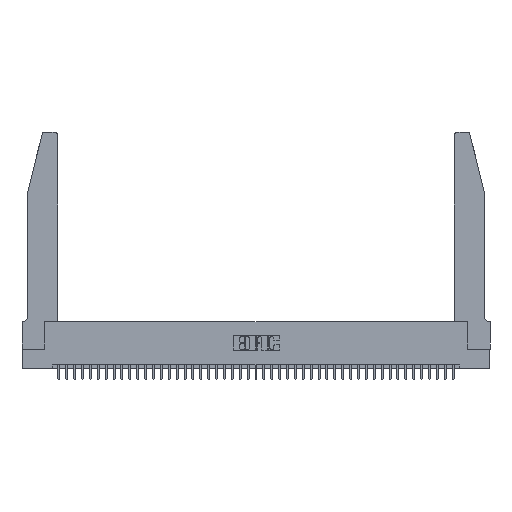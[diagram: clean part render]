
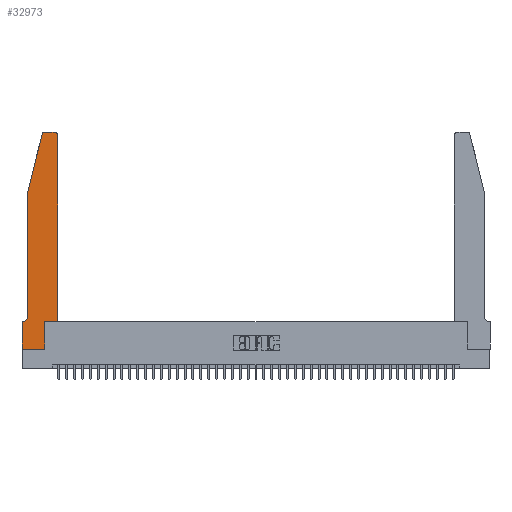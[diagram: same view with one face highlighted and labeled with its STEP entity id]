
A CAD part, top view. The second image highlights one B-rep face of the part: STEP entity #32973.
In plain terms, the highlighted planar face has unit normal (0, 0, 1).
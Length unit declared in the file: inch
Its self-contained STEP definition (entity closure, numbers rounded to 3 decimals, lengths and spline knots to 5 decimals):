
#164 = ORIENTED_EDGE ( 'NONE', *, *, #26499, .T. ) ;
#203 = ORIENTED_EDGE ( 'NONE', *, *, #35338, .T. ) ;
#878 = VERTEX_POINT ( 'NONE', #36373 ) ;
#2096 = LINE ( 'NONE', #17351, #25186 ) ;
#2854 = CARTESIAN_POINT ( 'NONE',  ( 0., 0.35, 0.37 ) ) ;
#3001 = VECTOR ( 'NONE', #38854, 39.37008 ) ;
#3074 = CARTESIAN_POINT ( 'NONE',  ( 0.2865, 0.35, 0.37 ) ) ;
#3281 = EDGE_CURVE ( 'NONE', #15961, #9850, #2096, .T. ) ;
#3304 = CARTESIAN_POINT ( 'NONE',  ( 0.0055, 0.42, 0.37 ) ) ;
#3636 = DIRECTION ( 'NONE',  ( -1., 0., 0. ) ) ;
#3750 = CARTESIAN_POINT ( 'NONE',  ( 0.4505, 0.35, 0.37 ) ) ;
#4304 = VERTEX_POINT ( 'NONE', #29953 ) ;
#4739 = DIRECTION ( 'NONE',  ( -0.239, -0.971, 0. ) ) ;
#4742 = DIRECTION ( 'NONE',  ( 1., 0., 0. ) ) ;
#5347 = DIRECTION ( 'NONE',  ( 0., 0., 1. ) ) ;
#5674 = VERTEX_POINT ( 'NONE', #12867 ) ;
#6853 = ORIENTED_EDGE ( 'NONE', *, *, #35453, .T. ) ;
#6986 = CARTESIAN_POINT ( 'NONE',  ( 0.0755, 0.35, 0.37 ) ) ;
#7164 = CARTESIAN_POINT ( 'NONE',  ( 0.0055, 0.35, 0.37 ) ) ;
#7631 = DIRECTION ( 'NONE',  ( 0., 0., 1. ) ) ;
#7651 = ORIENTED_EDGE ( 'NONE', *, *, #23992, .T. ) ;
#7680 = CIRCLE ( 'NONE', #9262, 0.07 ) ;
#8146 = EDGE_LOOP ( 'NONE', ( #14916, #164, #42248, #7651, #203, #36107, #33491, #30546, #33641, #6853, #37610, #27433 ) ) ;
#8549 = CIRCLE ( 'NONE', #38478, 0.03 ) ;
#9124 = EDGE_CURVE ( 'NONE', #31547, #4304, #24415, .T. ) ;
#9262 = AXIS2_PLACEMENT_3D ( 'NONE', #3304, #26938, #19879 ) ;
#9484 = PLANE ( 'NONE',  #35426 ) ;
#9835 = VECTOR ( 'NONE', #3636, 39.37008 ) ;
#9850 = VERTEX_POINT ( 'NONE', #31235 ) ;
#11353 = LINE ( 'NONE', #6986, #9835 ) ;
#11433 = EDGE_CURVE ( 'NONE', #878, #14352, #15251, .T. ) ;
#11893 = VECTOR ( 'NONE', #27755, 39.37008 ) ;
#12841 = DIRECTION ( 'NONE',  ( 1., 0., 0. ) ) ;
#12867 = CARTESIAN_POINT ( 'NONE',  ( 0.4205, 2.75, 0.37 ) ) ;
#13540 = VERTEX_POINT ( 'NONE', #7164 ) ;
#14352 = VERTEX_POINT ( 'NONE', #3074 ) ;
#14630 = EDGE_CURVE ( 'NONE', #13540, #31547, #11353, .T. ) ;
#14916 = ORIENTED_EDGE ( 'NONE', *, *, #17537, .T. ) ;
#15235 = CARTESIAN_POINT ( 'NONE',  ( 0.0755, 2., 0.37 ) ) ;
#15251 = LINE ( 'NONE', #27274, #16311 ) ;
#15961 = VERTEX_POINT ( 'NONE', #27917 ) ;
#16311 = VECTOR ( 'NONE', #17392, 39.37008 ) ;
#16482 = DIRECTION ( 'NONE',  ( -1., 0., 0. ) ) ;
#17351 = CARTESIAN_POINT ( 'NONE',  ( 0.0755, 2., 0.37 ) ) ;
#17392 = DIRECTION ( 'NONE',  ( 0., 1., 0. ) ) ;
#17537 = EDGE_CURVE ( 'NONE', #5674, #27048, #27216, .T. ) ;
#17990 = VERTEX_POINT ( 'NONE', #25415 ) ;
#18082 = CARTESIAN_POINT ( 'NONE',  ( 0., 0., 0.37 ) ) ;
#18446 = CARTESIAN_POINT ( 'NONE',  ( 0.284, 2.75, 0.37 ) ) ;
#19879 = DIRECTION ( 'NONE',  ( -1., 0., 0. ) ) ;
#20859 = LINE ( 'NONE', #15235, #3001 ) ;
#21325 = LINE ( 'NONE', #18082, #31338 ) ;
#21702 = FACE_OUTER_BOUND ( 'NONE', #8146, .T. ) ;
#21799 = DIRECTION ( 'NONE',  ( 1., 0., 0. ) ) ;
#23372 = LINE ( 'NONE', #3750, #24894 ) ;
#23623 = DIRECTION ( 'NONE',  ( 0., -1., 0. ) ) ;
#23992 = EDGE_CURVE ( 'NONE', #9850, #24051, #20859, .T. ) ;
#24051 = VERTEX_POINT ( 'NONE', #29260 ) ;
#24415 = LINE ( 'NONE', #29963, #24943 ) ;
#24791 = DIRECTION ( 'NONE',  ( 1., 0., 0. ) ) ;
#24894 = VECTOR ( 'NONE', #40127, 39.37008 ) ;
#24943 = VECTOR ( 'NONE', #23623, 39.37008 ) ;
#25186 = VECTOR ( 'NONE', #4739, 39.37008 ) ;
#25415 = CARTESIAN_POINT ( 'NONE',  ( 0.4505, 2.72, 0.37 ) ) ;
#25465 = CARTESIAN_POINT ( 'NONE',  ( 0.284, 2.72, 0.37 ) ) ;
#26050 = DIRECTION ( 'NONE',  ( 0., 0., 1. ) ) ;
#26499 = EDGE_CURVE ( 'NONE', #27048, #15961, #8549, .T. ) ;
#26938 = DIRECTION ( 'NONE',  ( 0., 0., -1. ) ) ;
#27048 = VERTEX_POINT ( 'NONE', #18446 ) ;
#27216 = LINE ( 'NONE', #33439, #32474 ) ;
#27274 = CARTESIAN_POINT ( 'NONE',  ( 0.2865, 0.35, 0.37 ) ) ;
#27433 = ORIENTED_EDGE ( 'NONE', *, *, #39938, .T. ) ;
#27755 = DIRECTION ( 'NONE',  ( 0., 1., 0. ) ) ;
#27917 = CARTESIAN_POINT ( 'NONE',  ( 0.25487, 2.72718, 0.37 ) ) ;
#28022 = CIRCLE ( 'NONE', #42927, 0.03 ) ;
#28630 = CARTESIAN_POINT ( 'NONE',  ( 0.4505, 0.35, 0.37 ) ) ;
#29260 = CARTESIAN_POINT ( 'NONE',  ( 0.0755, 0.42, 0.37 ) ) ;
#29831 = VERTEX_POINT ( 'NONE', #37114 ) ;
#29953 = CARTESIAN_POINT ( 'NONE',  ( 0., 0., 0.37 ) ) ;
#29963 = CARTESIAN_POINT ( 'NONE',  ( 0., 0., 0.37 ) ) ;
#30546 = ORIENTED_EDGE ( 'NONE', *, *, #43550, .T. ) ;
#31235 = CARTESIAN_POINT ( 'NONE',  ( 0.0755, 2., 0.37 ) ) ;
#31338 = VECTOR ( 'NONE', #4742, 39.37008 ) ;
#31547 = VERTEX_POINT ( 'NONE', #32951 ) ;
#32474 = VECTOR ( 'NONE', #16482, 39.37008 ) ;
#32951 = CARTESIAN_POINT ( 'NONE',  ( 0., 0.35, 0.37 ) ) ;
#32973 = ADVANCED_FACE ( 'NONE', ( #21702 ), #9484, .T. ) ;
#33439 = CARTESIAN_POINT ( 'NONE',  ( 0.2605, 2.75, 0.37 ) ) ;
#33491 = ORIENTED_EDGE ( 'NONE', *, *, #9124, .T. ) ;
#33641 = ORIENTED_EDGE ( 'NONE', *, *, #11433, .T. ) ;
#34981 = CARTESIAN_POINT ( 'NONE',  ( 0.4205, 2.72, 0.37 ) ) ;
#35338 = EDGE_CURVE ( 'NONE', #24051, #13540, #7680, .T. ) ;
#35426 = AXIS2_PLACEMENT_3D ( 'NONE', #2854, #26050, #12841 ) ;
#35453 = EDGE_CURVE ( 'NONE', #14352, #29831, #23372, .T. ) ;
#36107 = ORIENTED_EDGE ( 'NONE', *, *, #14630, .T. ) ;
#36373 = CARTESIAN_POINT ( 'NONE',  ( 0.2865, 0., 0.37 ) ) ;
#36949 = EDGE_CURVE ( 'NONE', #29831, #17990, #41432, .T. ) ;
#37114 = CARTESIAN_POINT ( 'NONE',  ( 0.4505, 0.35, 0.37 ) ) ;
#37610 = ORIENTED_EDGE ( 'NONE', *, *, #36949, .T. ) ;
#38478 = AXIS2_PLACEMENT_3D ( 'NONE', #25465, #5347, #21799 ) ;
#38854 = DIRECTION ( 'NONE',  ( 0., -1., 0. ) ) ;
#39938 = EDGE_CURVE ( 'NONE', #17990, #5674, #28022, .T. ) ;
#40127 = DIRECTION ( 'NONE',  ( 1., 0., 0. ) ) ;
#41432 = LINE ( 'NONE', #28630, #11893 ) ;
#42248 = ORIENTED_EDGE ( 'NONE', *, *, #3281, .T. ) ;
#42927 = AXIS2_PLACEMENT_3D ( 'NONE', #34981, #7631, #24791 ) ;
#43550 = EDGE_CURVE ( 'NONE', #4304, #878, #21325, .T. ) ;
